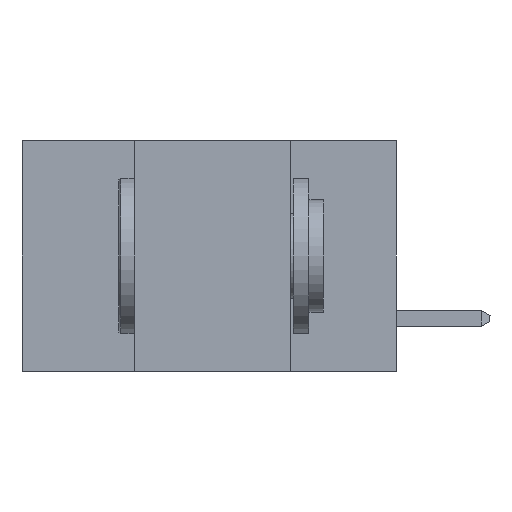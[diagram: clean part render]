
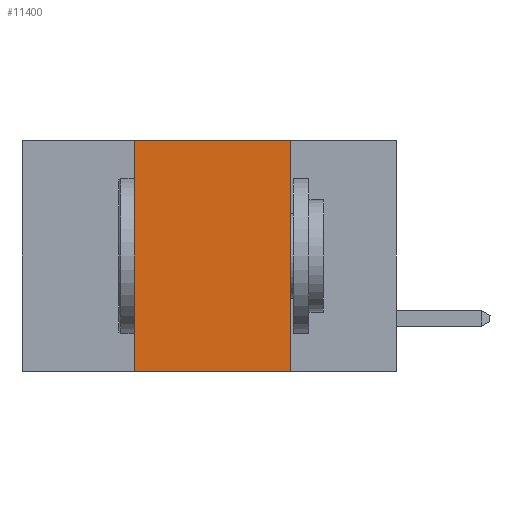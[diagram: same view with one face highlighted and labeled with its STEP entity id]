
A CAD part, left-side view. The second image highlights one B-rep face of the part: STEP entity #11400.
In plain terms, the highlighted planar face has unit normal (-1, 0, 0).
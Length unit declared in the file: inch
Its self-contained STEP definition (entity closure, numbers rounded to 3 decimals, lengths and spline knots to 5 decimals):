
#164 = VECTOR ( 'NONE', #16171, 39.37008 ) ;
#173 = CARTESIAN_POINT ( 'NONE',  ( 0., 0.6, 0. ) ) ;
#1390 = EDGE_CURVE ( 'NONE', #8811, #19449, #3443, .T. ) ;
#1810 = DIRECTION ( 'NONE',  ( 0., 0., 1. ) ) ;
#2549 = CARTESIAN_POINT ( 'NONE',  ( 0., 0.17, -0.37 ) ) ;
#3118 = LINE ( 'NONE', #8134, #12996 ) ;
#3188 = AXIS2_PLACEMENT_3D ( 'NONE', #9464, #7930, #4560 ) ;
#3443 = LINE ( 'NONE', #173, #9950 ) ;
#3573 = CARTESIAN_POINT ( 'NONE',  ( 0., 0.17, 0. ) ) ;
#4560 = DIRECTION ( 'NONE',  ( 0., 0., -1. ) ) ;
#4758 = FACE_OUTER_BOUND ( 'NONE', #7536, .T. ) ;
#4832 = VERTEX_POINT ( 'NONE', #2549 ) ;
#5504 = ORIENTED_EDGE ( 'NONE', *, *, #1390, .F. ) ;
#6719 = LINE ( 'NONE', #9495, #13096 ) ;
#7536 = EDGE_LOOP ( 'NONE', ( #10652, #5504, #19625, #16998 ) ) ;
#7719 = DIRECTION ( 'NONE',  ( 0., 0., -1. ) ) ;
#7930 = DIRECTION ( 'NONE',  ( 1., 0., 0. ) ) ;
#8134 = CARTESIAN_POINT ( 'NONE',  ( 0., 0.17, -0.37 ) ) ;
#8389 = CARTESIAN_POINT ( 'NONE',  ( 0., 0.6, -0.37 ) ) ;
#8420 = EDGE_CURVE ( 'NONE', #17349, #4832, #19635, .T. ) ;
#8811 = VERTEX_POINT ( 'NONE', #16147 ) ;
#9464 = CARTESIAN_POINT ( 'NONE',  ( 0., 0.6, 0. ) ) ;
#9495 = CARTESIAN_POINT ( 'NONE',  ( 0., 0.42, -0.37 ) ) ;
#9950 = VECTOR ( 'NONE', #12665, 39.37008 ) ;
#10652 = ORIENTED_EDGE ( 'NONE', *, *, #11283, .F. ) ;
#10990 = PLANE ( 'NONE',  #3188 ) ;
#11283 = EDGE_CURVE ( 'NONE', #19449, #4832, #3118, .T. ) ;
#11400 = ADVANCED_FACE ( 'NONE', ( #4758 ), #10990, .F. ) ;
#12665 = DIRECTION ( 'NONE',  ( 0., -1., 0. ) ) ;
#12996 = VECTOR ( 'NONE', #7719, 39.37008 ) ;
#13096 = VECTOR ( 'NONE', #1810, 39.37008 ) ;
#16147 = CARTESIAN_POINT ( 'NONE',  ( 0., 0.42, 0. ) ) ;
#16171 = DIRECTION ( 'NONE',  ( 0., -1., 0. ) ) ;
#16754 = EDGE_CURVE ( 'NONE', #17349, #8811, #6719, .T. ) ;
#16998 = ORIENTED_EDGE ( 'NONE', *, *, #8420, .T. ) ;
#17349 = VERTEX_POINT ( 'NONE', #18230 ) ;
#18230 = CARTESIAN_POINT ( 'NONE',  ( 0., 0.42, -0.37 ) ) ;
#19449 = VERTEX_POINT ( 'NONE', #3573 ) ;
#19625 = ORIENTED_EDGE ( 'NONE', *, *, #16754, .F. ) ;
#19635 = LINE ( 'NONE', #8389, #164 ) ;
